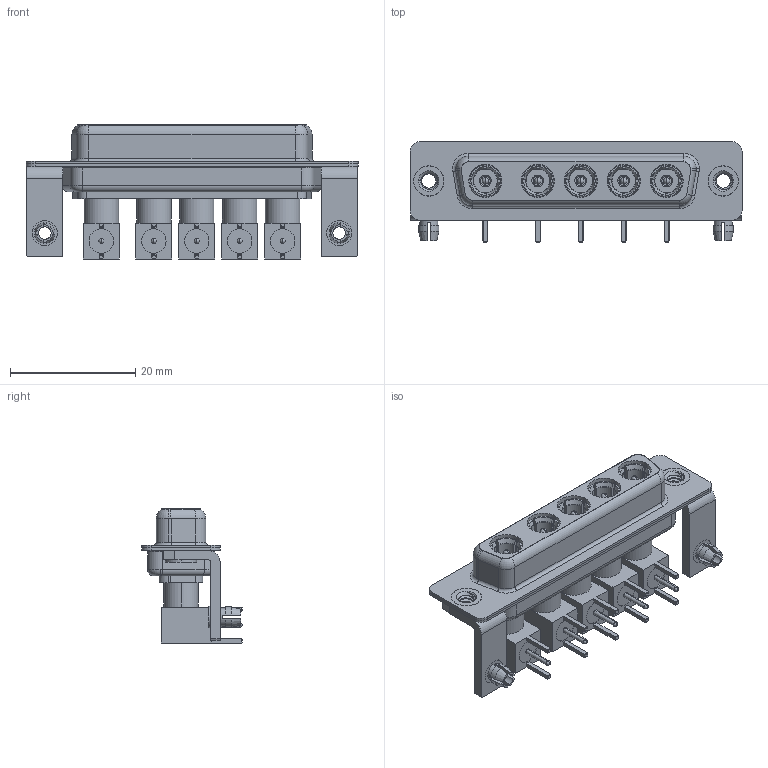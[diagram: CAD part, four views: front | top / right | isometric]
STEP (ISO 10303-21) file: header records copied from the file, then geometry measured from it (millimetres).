
FILE_DESCRIPTION (( 'STEP AP203' ), '1' );
FILE_NAME ('630-5W5-240-7T3.STEP', '2022-05-31T22:17:13', ( '' ), ( '' ), 'SwSTEP 2.0', 'SolidWorks 2020', '' );
FILE_SCHEMA (( 'CONFIG_CONTROL_DESIGN' ));
Length unit declared in the file: millimetre
Products named in the file (18): Co-Ax Plug Assy_RA; Pin_RA; RA Back Shell; Insulator Pin_Straight PC Tail; Co-Ax Plug_RA PC Tail; 630Combo Stabilizer Bracket; Locking Collar; 630-5W5-240-7T3; 630Combo Shell Front_25 Contacts; 630Combo Shell Rear_25 Contacts; 630Combo Housing_5W5; 630Combo Threaded Rivet_3; 630Combo Board Lock; Insulator RA Pin
Assembly tree (44 placements, depth 3):
  630-5W5-240-7T3
    630Combo Housing_5W5
    630Combo Shell Front_25 Contacts
    630Combo Shell Rear_25 Contacts
    630Combo Threaded Rivet_3  x2
    630Combo Stabilizer Bracket  x2
    630Combo Board Lock  x2
    Co-Ax Plug Assy_RA
      Co-Ax Plug_RA PC Tail
      Insulator Pin_Straight PC Tail
      Pin_RA
      Locking Collar
      RA Back Shell
      Insulator RA Pin
    Co-Ax Plug Assy_RA
      Co-Ax Plug_RA PC Tail
      Insulator Pin_Straight PC Tail
      Pin_RA
      Locking Collar
      RA Back Shell
      Insulator RA Pin
    Co-Ax Plug Assy_RA
      Co-Ax Plug_RA PC Tail
      Insulator Pin_Straight PC Tail
      Pin_RA
      Locking Collar
      RA Back Shell
      Insulator RA Pin
    Co-Ax Plug Assy_RA
      Co-Ax Plug_RA PC Tail
      Insulator Pin_Straight PC Tail
      Pin_RA
      Locking Collar
      RA Back Shell
      Insulator RA Pin
    Co-Ax Plug Assy_RA
      Co-Ax Plug_RA PC Tail
      Insulator Pin_Straight PC Tail
      Pin_RA
      Locking Collar
      RA Back Shell
      Insulator RA Pin
Bounding box: 53.05 x 16 x 21.41 mm (x, y, z)
Volume: 5156.4 mm3; surface area: 12592.2 mm2
Topology: 39 solids, 39 shells, 1251 faces, 3040 edges, 1912 vertices
Faces by surface type: cylinder 512, plane 470, cone 151, torus 87, sphere 20, bspline 11
Entity records: 19273 total; most frequent: CARTESIAN_POINT 4420, DIRECTION 2772, ORIENTED_EDGE 2432, EDGE_CURVE 1216, AXIS2_PLACEMENT_3D 1113, VERTEX_POINT 771, EDGE_LOOP 569, CIRCLE 565
